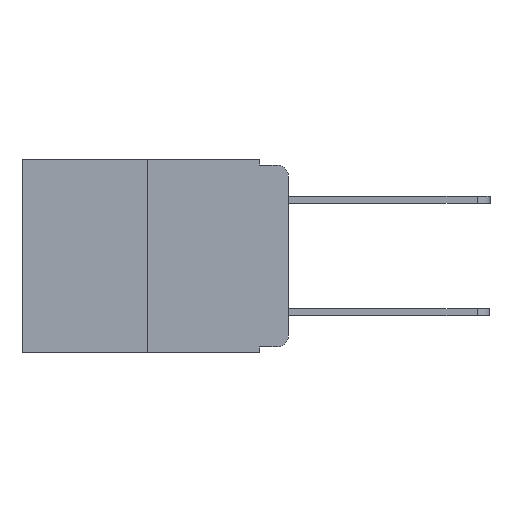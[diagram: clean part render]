
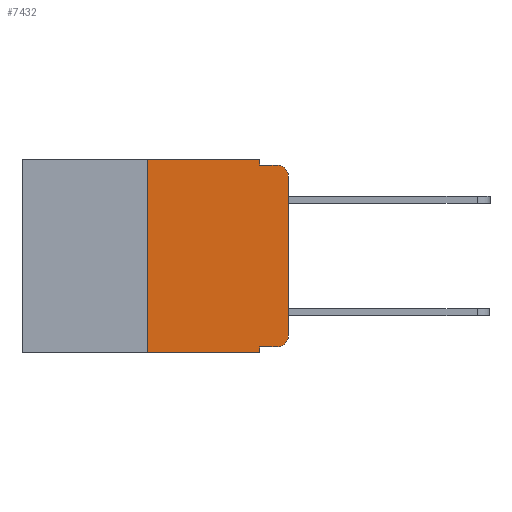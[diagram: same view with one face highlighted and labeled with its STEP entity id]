
A CAD part, left-side view. The second image highlights one B-rep face of the part: STEP entity #7432.
In plain terms, the highlighted planar face has unit normal (-1, 0, 0).
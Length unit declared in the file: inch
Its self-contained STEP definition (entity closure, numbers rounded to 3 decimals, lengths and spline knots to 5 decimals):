
#166 = ORIENTED_EDGE ( 'NONE', *, *, #15256, .F. ) ;
#686 = VERTEX_POINT ( 'NONE', #21804 ) ;
#839 = EDGE_CURVE ( 'NONE', #10597, #13081, #17453, .T. ) ;
#1283 = LINE ( 'NONE', #4788, #15773 ) ;
#1560 = ORIENTED_EDGE ( 'NONE', *, *, #839, .T. ) ;
#2226 = VECTOR ( 'NONE', #2575, 39.37008 ) ;
#2330 = VERTEX_POINT ( 'NONE', #13962 ) ;
#2523 = ORIENTED_EDGE ( 'NONE', *, *, #10217, .T. ) ;
#2528 = CARTESIAN_POINT ( 'NONE',  ( 0., 0.473, 0. ) ) ;
#2575 = DIRECTION ( 'NONE',  ( 0., 0., -1. ) ) ;
#2699 = DIRECTION ( 'NONE',  ( 0., -1., 0. ) ) ;
#2761 = DIRECTION ( 'NONE',  ( 0., 0., -1. ) ) ;
#2816 = CIRCLE ( 'NONE', #23231, 0.02 ) ;
#3636 = VECTOR ( 'NONE', #2699, 39.37008 ) ;
#4386 = CARTESIAN_POINT ( 'NONE',  ( 0., 0.25, 0. ) ) ;
#4415 = DIRECTION ( 'NONE',  ( 0., -1., 0. ) ) ;
#4715 = CARTESIAN_POINT ( 'NONE',  ( 0., 0., -0.313 ) ) ;
#4788 = CARTESIAN_POINT ( 'NONE',  ( 0., 0., 0. ) ) ;
#5131 = LINE ( 'NONE', #2528, #9566 ) ;
#5134 = EDGE_CURVE ( 'NONE', #2330, #8096, #2816, .T. ) ;
#5761 = CARTESIAN_POINT ( 'NONE',  ( 0., 0.02, -0.313 ) ) ;
#5967 = EDGE_LOOP ( 'NONE', ( #23553, #1560, #20178, #21854, #17265, #166, #13342, #9016, #2523, #6446 ) ) ;
#6446 = ORIENTED_EDGE ( 'NONE', *, *, #5134, .T. ) ;
#6703 = DIRECTION ( 'NONE',  ( 0., 0., 1. ) ) ;
#7160 = LINE ( 'NONE', #4386, #21468 ) ;
#7432 = ADVANCED_FACE ( 'NONE', ( #14819 ), #23306, .F. ) ;
#7680 = DIRECTION ( 'NONE',  ( 0., 0., -1. ) ) ;
#8096 = VERTEX_POINT ( 'NONE', #4715 ) ;
#8416 = CARTESIAN_POINT ( 'NONE',  ( 0., 0.473, -0.343 ) ) ;
#9016 = ORIENTED_EDGE ( 'NONE', *, *, #11477, .F. ) ;
#9390 = VECTOR ( 'NONE', #12294, 39.37008 ) ;
#9566 = VECTOR ( 'NONE', #4415, 39.37008 ) ;
#10127 = LINE ( 'NONE', #12277, #19504 ) ;
#10217 = EDGE_CURVE ( 'NONE', #686, #2330, #19381, .T. ) ;
#10408 = CARTESIAN_POINT ( 'NONE',  ( 0., 0.051, -0.333 ) ) ;
#10597 = VERTEX_POINT ( 'NONE', #18904 ) ;
#11477 = EDGE_CURVE ( 'NONE', #686, #16848, #22742, .T. ) ;
#11857 = LINE ( 'NONE', #13666, #21168 ) ;
#12006 = CARTESIAN_POINT ( 'NONE',  ( 0., 0.051, 0. ) ) ;
#12196 = CARTESIAN_POINT ( 'NONE',  ( 0., 0.473, 0. ) ) ;
#12277 = CARTESIAN_POINT ( 'NONE',  ( 0., 0.051, -0.01 ) ) ;
#12294 = DIRECTION ( 'NONE',  ( 0., -1., 0. ) ) ;
#13081 = VERTEX_POINT ( 'NONE', #24190 ) ;
#13281 = CARTESIAN_POINT ( 'NONE',  ( 0., 0.051, -0.01 ) ) ;
#13342 = ORIENTED_EDGE ( 'NONE', *, *, #23321, .T. ) ;
#13565 = EDGE_CURVE ( 'NONE', #21316, #14873, #5131, .T. ) ;
#13666 = CARTESIAN_POINT ( 'NONE',  ( 0., 0.051, 0. ) ) ;
#13962 = CARTESIAN_POINT ( 'NONE',  ( 0., 0.02, -0.333 ) ) ;
#14081 = DIRECTION ( 'NONE',  ( 1., 0., 0. ) ) ;
#14160 = DIRECTION ( 'NONE',  ( 0., -1., 0. ) ) ;
#14172 = DIRECTION ( 'NONE',  ( 0., 0., -1. ) ) ;
#14791 = AXIS2_PLACEMENT_3D ( 'NONE', #21545, #19192, #14172 ) ;
#14819 = FACE_OUTER_BOUND ( 'NONE', #5967, .T. ) ;
#14873 = VERTEX_POINT ( 'NONE', #20096 ) ;
#15256 = EDGE_CURVE ( 'NONE', #21304, #21316, #7160, .T. ) ;
#15554 = DIRECTION ( 'NONE',  ( 0., 0., -1. ) ) ;
#15698 = DIRECTION ( 'NONE',  ( 0., 0., 1. ) ) ;
#15773 = VECTOR ( 'NONE', #6703, 39.37008 ) ;
#16848 = VERTEX_POINT ( 'NONE', #20316 ) ;
#17265 = ORIENTED_EDGE ( 'NONE', *, *, #13565, .F. ) ;
#17288 = EDGE_CURVE ( 'NONE', #8096, #10597, #1283, .T. ) ;
#17453 = CIRCLE ( 'NONE', #14791, 0.02 ) ;
#18064 = LINE ( 'NONE', #8416, #3636 ) ;
#18660 = AXIS2_PLACEMENT_3D ( 'NONE', #12196, #14081, #2761 ) ;
#18904 = CARTESIAN_POINT ( 'NONE',  ( 0., 0., -0.03 ) ) ;
#18912 = DIRECTION ( 'NONE',  ( -1., 0., 0. ) ) ;
#19000 = EDGE_CURVE ( 'NONE', #14873, #20104, #11857, .T. ) ;
#19192 = DIRECTION ( 'NONE',  ( -1., 0., 0. ) ) ;
#19255 = CARTESIAN_POINT ( 'NONE',  ( 0., 0.25, -0.343 ) ) ;
#19327 = CARTESIAN_POINT ( 'NONE',  ( 0., 0.25, 0. ) ) ;
#19381 = LINE ( 'NONE', #10408, #9390 ) ;
#19504 = VECTOR ( 'NONE', #14160, 39.37008 ) ;
#20096 = CARTESIAN_POINT ( 'NONE',  ( 0., 0.051, 0. ) ) ;
#20104 = VERTEX_POINT ( 'NONE', #13281 ) ;
#20178 = ORIENTED_EDGE ( 'NONE', *, *, #23920, .F. ) ;
#20316 = CARTESIAN_POINT ( 'NONE',  ( 0., 0.051, -0.343 ) ) ;
#21168 = VECTOR ( 'NONE', #15554, 39.37008 ) ;
#21304 = VERTEX_POINT ( 'NONE', #19255 ) ;
#21316 = VERTEX_POINT ( 'NONE', #19327 ) ;
#21468 = VECTOR ( 'NONE', #15698, 39.37008 ) ;
#21545 = CARTESIAN_POINT ( 'NONE',  ( 0., 0.02, -0.03 ) ) ;
#21804 = CARTESIAN_POINT ( 'NONE',  ( 0., 0.051, -0.333 ) ) ;
#21854 = ORIENTED_EDGE ( 'NONE', *, *, #19000, .F. ) ;
#22742 = LINE ( 'NONE', #12006, #2226 ) ;
#23231 = AXIS2_PLACEMENT_3D ( 'NONE', #5761, #18912, #7680 ) ;
#23306 = PLANE ( 'NONE',  #18660 ) ;
#23321 = EDGE_CURVE ( 'NONE', #21304, #16848, #18064, .T. ) ;
#23553 = ORIENTED_EDGE ( 'NONE', *, *, #17288, .T. ) ;
#23920 = EDGE_CURVE ( 'NONE', #20104, #13081, #10127, .T. ) ;
#24190 = CARTESIAN_POINT ( 'NONE',  ( 0., 0.02, -0.01 ) ) ;
